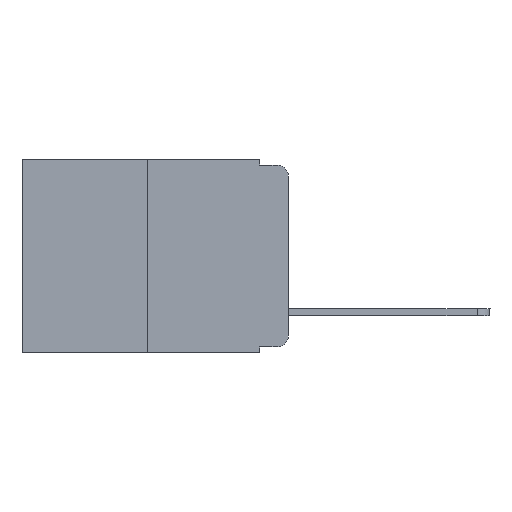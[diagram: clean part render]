
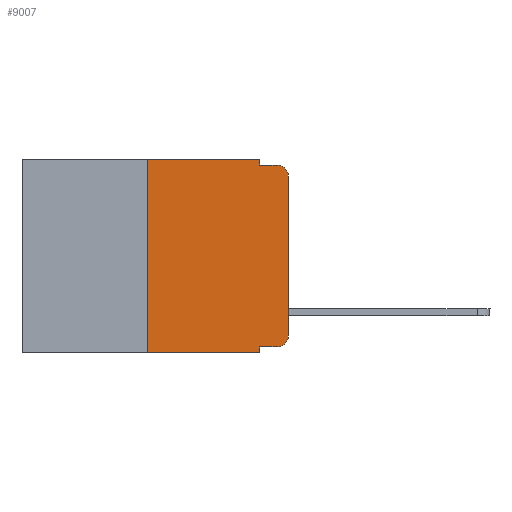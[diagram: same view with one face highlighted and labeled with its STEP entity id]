
A CAD part, left-side view. The second image highlights one B-rep face of the part: STEP entity #9007.
In plain terms, the highlighted planar face has unit normal (-1, 0, 0).
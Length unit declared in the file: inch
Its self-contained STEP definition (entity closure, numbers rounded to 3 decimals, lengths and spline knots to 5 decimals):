
#4 = ORIENTED_EDGE ( 'NONE', *, *, #13865, .T. ) ;
#295 = CARTESIAN_POINT ( 'NONE',  ( 0., 0.051, -0.333 ) ) ;
#687 = ORIENTED_EDGE ( 'NONE', *, *, #6323, .F. ) ;
#845 = CARTESIAN_POINT ( 'NONE',  ( 0., 0., -0.313 ) ) ;
#974 = DIRECTION ( 'NONE',  ( 0., 0., -1. ) ) ;
#988 = DIRECTION ( 'NONE',  ( -1., 0., 0. ) ) ;
#1226 = VECTOR ( 'NONE', #7781, 39.37008 ) ;
#1308 = DIRECTION ( 'NONE',  ( -1., 0., 0. ) ) ;
#1355 = VERTEX_POINT ( 'NONE', #12843 ) ;
#1408 = FACE_OUTER_BOUND ( 'NONE', #2892, .T. ) ;
#1620 = CARTESIAN_POINT ( 'NONE',  ( 0., 0.473, 0. ) ) ;
#1635 = VERTEX_POINT ( 'NONE', #9349 ) ;
#2251 = CARTESIAN_POINT ( 'NONE',  ( 0., 0.25, -0.343 ) ) ;
#2603 = DIRECTION ( 'NONE',  ( 1., 0., 0. ) ) ;
#2767 = ORIENTED_EDGE ( 'NONE', *, *, #4182, .T. ) ;
#2892 = EDGE_LOOP ( 'NONE', ( #7252, #4788, #687, #11850, #4863, #3183, #5098, #4248, #4, #2767 ) ) ;
#3047 = VERTEX_POINT ( 'NONE', #5509 ) ;
#3134 = CARTESIAN_POINT ( 'NONE',  ( 0., 0.473, 0. ) ) ;
#3139 = CARTESIAN_POINT ( 'NONE',  ( 0., 0.02, -0.03 ) ) ;
#3183 = ORIENTED_EDGE ( 'NONE', *, *, #12851, .F. ) ;
#3474 = DIRECTION ( 'NONE',  ( 0., -1., 0. ) ) ;
#3552 = VECTOR ( 'NONE', #13277, 39.37008 ) ;
#3607 = CARTESIAN_POINT ( 'NONE',  ( 0., 0.473, -0.343 ) ) ;
#4182 = EDGE_CURVE ( 'NONE', #3047, #5733, #11830, .T. ) ;
#4248 = ORIENTED_EDGE ( 'NONE', *, *, #7036, .F. ) ;
#4344 = EDGE_CURVE ( 'NONE', #7486, #6051, #10257, .T. ) ;
#4595 = LINE ( 'NONE', #295, #11669 ) ;
#4642 = AXIS2_PLACEMENT_3D ( 'NONE', #10642, #988, #7390 ) ;
#4751 = LINE ( 'NONE', #3607, #5786 ) ;
#4788 = ORIENTED_EDGE ( 'NONE', *, *, #4344, .T. ) ;
#4863 = ORIENTED_EDGE ( 'NONE', *, *, #13287, .F. ) ;
#5084 = DIRECTION ( 'NONE',  ( 0., 0., 1. ) ) ;
#5098 = ORIENTED_EDGE ( 'NONE', *, *, #11633, .T. ) ;
#5161 = CARTESIAN_POINT ( 'NONE',  ( 0., 0.25, 0. ) ) ;
#5509 = CARTESIAN_POINT ( 'NONE',  ( 0., 0.02, -0.333 ) ) ;
#5547 = AXIS2_PLACEMENT_3D ( 'NONE', #3139, #1308, #11872 ) ;
#5733 = VERTEX_POINT ( 'NONE', #845 ) ;
#5780 = VECTOR ( 'NONE', #12189, 39.37008 ) ;
#5786 = VECTOR ( 'NONE', #3474, 39.37008 ) ;
#5933 = DIRECTION ( 'NONE',  ( 0., 0., -1. ) ) ;
#6051 = VERTEX_POINT ( 'NONE', #10408 ) ;
#6121 = CARTESIAN_POINT ( 'NONE',  ( 0., 0.051, 0. ) ) ;
#6323 = EDGE_CURVE ( 'NONE', #13443, #6051, #11145, .T. ) ;
#6337 = LINE ( 'NONE', #10628, #12048 ) ;
#6767 = PLANE ( 'NONE',  #10498 ) ;
#7036 = EDGE_CURVE ( 'NONE', #1355, #1635, #6337, .T. ) ;
#7252 = ORIENTED_EDGE ( 'NONE', *, *, #8985, .T. ) ;
#7348 = DIRECTION ( 'NONE',  ( 0., -1., 0. ) ) ;
#7390 = DIRECTION ( 'NONE',  ( 0., 0., -1. ) ) ;
#7486 = VERTEX_POINT ( 'NONE', #8360 ) ;
#7551 = VERTEX_POINT ( 'NONE', #12086 ) ;
#7711 = LINE ( 'NONE', #5161, #10970 ) ;
#7781 = DIRECTION ( 'NONE',  ( 0., 0., -1. ) ) ;
#7900 = CARTESIAN_POINT ( 'NONE',  ( 0., 0.051, -0.01 ) ) ;
#8360 = CARTESIAN_POINT ( 'NONE',  ( 0., 0., -0.03 ) ) ;
#8947 = DIRECTION ( 'NONE',  ( 0., -1., 0. ) ) ;
#8985 = EDGE_CURVE ( 'NONE', #5733, #7486, #9073, .T. ) ;
#9007 = ADVANCED_FACE ( 'NONE', ( #1408 ), #6767, .F. ) ;
#9073 = LINE ( 'NONE', #12129, #5780 ) ;
#9349 = CARTESIAN_POINT ( 'NONE',  ( 0., 0.051, -0.343 ) ) ;
#9883 = EDGE_CURVE ( 'NONE', #12492, #13443, #13356, .T. ) ;
#10094 = VECTOR ( 'NONE', #7348, 39.37008 ) ;
#10257 = CIRCLE ( 'NONE', #5547, 0.02 ) ;
#10408 = CARTESIAN_POINT ( 'NONE',  ( 0., 0.02, -0.01 ) ) ;
#10498 = AXIS2_PLACEMENT_3D ( 'NONE', #1620, #2603, #5933 ) ;
#10628 = CARTESIAN_POINT ( 'NONE',  ( 0., 0.051, 0. ) ) ;
#10642 = CARTESIAN_POINT ( 'NONE',  ( 0., 0.02, -0.313 ) ) ;
#10647 = VERTEX_POINT ( 'NONE', #2251 ) ;
#10970 = VECTOR ( 'NONE', #5084, 39.37008 ) ;
#11145 = LINE ( 'NONE', #7900, #3552 ) ;
#11156 = CARTESIAN_POINT ( 'NONE',  ( 0., 0.051, -0.01 ) ) ;
#11633 = EDGE_CURVE ( 'NONE', #10647, #1635, #4751, .T. ) ;
#11669 = VECTOR ( 'NONE', #8947, 39.37008 ) ;
#11830 = CIRCLE ( 'NONE', #4642, 0.02 ) ;
#11850 = ORIENTED_EDGE ( 'NONE', *, *, #9883, .F. ) ;
#11872 = DIRECTION ( 'NONE',  ( 0., 0., -1. ) ) ;
#11938 = LINE ( 'NONE', #3134, #10094 ) ;
#12048 = VECTOR ( 'NONE', #974, 39.37008 ) ;
#12086 = CARTESIAN_POINT ( 'NONE',  ( 0., 0.25, 0. ) ) ;
#12129 = CARTESIAN_POINT ( 'NONE',  ( 0., 0., 0. ) ) ;
#12159 = CARTESIAN_POINT ( 'NONE',  ( 0., 0.051, 0. ) ) ;
#12189 = DIRECTION ( 'NONE',  ( 0., 0., 1. ) ) ;
#12492 = VERTEX_POINT ( 'NONE', #6121 ) ;
#12843 = CARTESIAN_POINT ( 'NONE',  ( 0., 0.051, -0.333 ) ) ;
#12851 = EDGE_CURVE ( 'NONE', #10647, #7551, #7711, .T. ) ;
#13277 = DIRECTION ( 'NONE',  ( 0., -1., 0. ) ) ;
#13287 = EDGE_CURVE ( 'NONE', #7551, #12492, #11938, .T. ) ;
#13356 = LINE ( 'NONE', #12159, #1226 ) ;
#13443 = VERTEX_POINT ( 'NONE', #11156 ) ;
#13865 = EDGE_CURVE ( 'NONE', #1355, #3047, #4595, .T. ) ;
